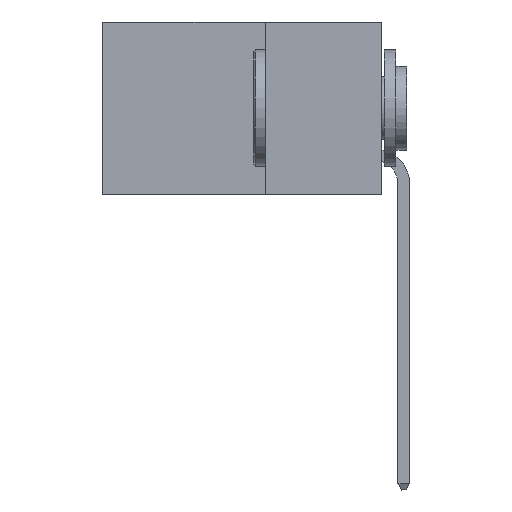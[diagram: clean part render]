
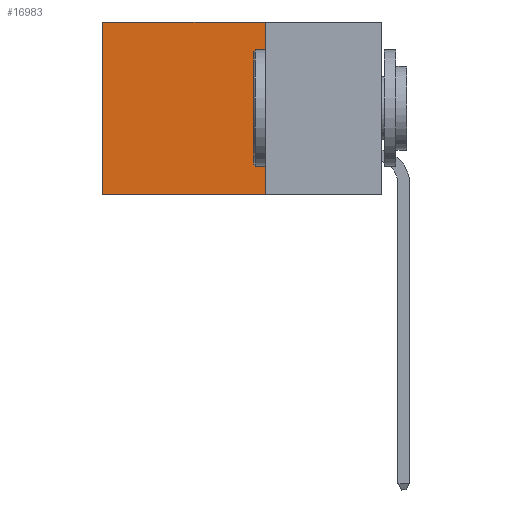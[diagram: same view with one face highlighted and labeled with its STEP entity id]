
A CAD part, left-side view. The second image highlights one B-rep face of the part: STEP entity #16983.
In plain terms, the highlighted planar face has unit normal (-1, 0, 0).
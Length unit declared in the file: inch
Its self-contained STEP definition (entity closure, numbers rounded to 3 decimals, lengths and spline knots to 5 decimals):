
#1930 = DIRECTION ( 'NONE',  ( 0., 0., -1. ) ) ;
#5149 = VECTOR ( 'NONE', #14342, 39.37008 ) ;
#5480 = FACE_OUTER_BOUND ( 'NONE', #26524, .T. ) ;
#6582 = LINE ( 'NONE', #28791, #19592 ) ;
#6681 = LINE ( 'NONE', #29393, #15252 ) ;
#7541 = CARTESIAN_POINT ( 'NONE',  ( 0.2875, 0.25, -0.37 ) ) ;
#8423 = LINE ( 'NONE', #32978, #23887 ) ;
#9631 = CARTESIAN_POINT ( 'NONE',  ( 0.2875, 0.25, 0. ) ) ;
#11619 = AXIS2_PLACEMENT_3D ( 'NONE', #9631, #33221, #1930 ) ;
#11628 = EDGE_CURVE ( 'NONE', #12060, #17220, #6681, .T. ) ;
#11957 = CARTESIAN_POINT ( 'NONE',  ( 0.2875, 0.25, 0. ) ) ;
#12060 = VERTEX_POINT ( 'NONE', #7541 ) ;
#14342 = DIRECTION ( 'NONE',  ( 0., 0., -1. ) ) ;
#15252 = VECTOR ( 'NONE', #16433, 39.37008 ) ;
#16433 = DIRECTION ( 'NONE',  ( 0., 1., 0. ) ) ;
#16983 = ADVANCED_FACE ( 'NONE', ( #5480 ), #20366, .F. ) ;
#17220 = VERTEX_POINT ( 'NONE', #28965 ) ;
#18590 = DIRECTION ( 'NONE',  ( 0., 0., -1. ) ) ;
#18944 = VERTEX_POINT ( 'NONE', #27398 ) ;
#19592 = VECTOR ( 'NONE', #18590, 39.37008 ) ;
#19759 = EDGE_CURVE ( 'NONE', #18944, #17220, #6582, .T. ) ;
#20366 = PLANE ( 'NONE',  #11619 ) ;
#20670 = EDGE_CURVE ( 'NONE', #24864, #18944, #8423, .T. ) ;
#23887 = VECTOR ( 'NONE', #27782, 39.37008 ) ;
#24530 = CARTESIAN_POINT ( 'NONE',  ( 0.2875, 0.25, 0. ) ) ;
#24864 = VERTEX_POINT ( 'NONE', #24530 ) ;
#25124 = ORIENTED_EDGE ( 'NONE', *, *, #11628, .F. ) ;
#26524 = EDGE_LOOP ( 'NONE', ( #30465, #25124, #26843, #27133 ) ) ;
#26779 = EDGE_CURVE ( 'NONE', #24864, #12060, #27920, .T. ) ;
#26843 = ORIENTED_EDGE ( 'NONE', *, *, #26779, .F. ) ;
#27133 = ORIENTED_EDGE ( 'NONE', *, *, #20670, .T. ) ;
#27398 = CARTESIAN_POINT ( 'NONE',  ( 0.2875, 0.6, 0. ) ) ;
#27782 = DIRECTION ( 'NONE',  ( 0., 1., 0. ) ) ;
#27920 = LINE ( 'NONE', #11957, #5149 ) ;
#28791 = CARTESIAN_POINT ( 'NONE',  ( 0.2875, 0.6, 0. ) ) ;
#28965 = CARTESIAN_POINT ( 'NONE',  ( 0.2875, 0.6, -0.37 ) ) ;
#29393 = CARTESIAN_POINT ( 'NONE',  ( 0.2875, 0.25, -0.37 ) ) ;
#30465 = ORIENTED_EDGE ( 'NONE', *, *, #19759, .T. ) ;
#32978 = CARTESIAN_POINT ( 'NONE',  ( 0.2875, 0.25, 0. ) ) ;
#33221 = DIRECTION ( 'NONE',  ( 1., 0., 0. ) ) ;
